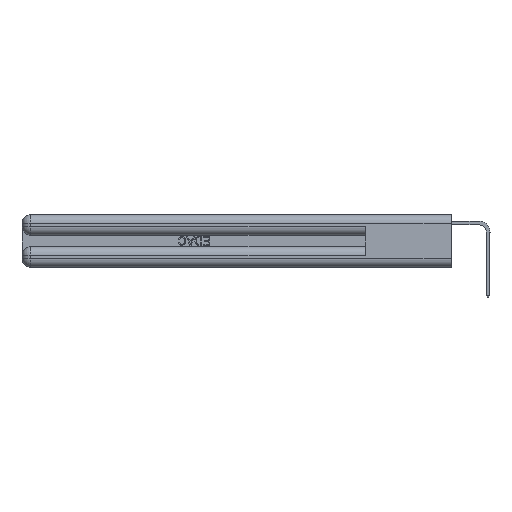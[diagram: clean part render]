
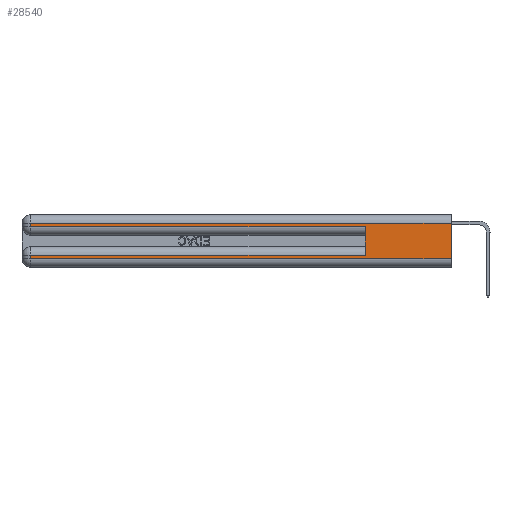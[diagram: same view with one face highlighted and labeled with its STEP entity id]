
A CAD part, left-side view. The second image highlights one B-rep face of the part: STEP entity #28540.
In plain terms, the highlighted planar face has unit normal (-1, 0, 0).
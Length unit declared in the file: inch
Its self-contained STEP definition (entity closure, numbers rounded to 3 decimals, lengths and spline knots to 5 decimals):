
#274 = DIRECTION ( 'NONE',  ( 0., 0., 1. ) ) ;
#744 = CARTESIAN_POINT ( 'NONE',  ( 0., 0., 0.06 ) ) ;
#1285 = EDGE_CURVE ( 'NONE', #16184, #5448, #23620, .T. ) ;
#1514 = LINE ( 'NONE', #28508, #15376 ) ;
#1540 = VECTOR ( 'NONE', #11069, 39.37008 ) ;
#1986 = VECTOR ( 'NONE', #16828, 39.37008 ) ;
#2475 = CARTESIAN_POINT ( 'NONE',  ( 0., 2.94, 0.37 ) ) ;
#2780 = CARTESIAN_POINT ( 'NONE',  ( 0., 0., 0.285 ) ) ;
#2801 = LINE ( 'NONE', #14213, #1986 ) ;
#3840 = LINE ( 'NONE', #744, #9959 ) ;
#4921 = LINE ( 'NONE', #2780, #11020 ) ;
#5448 = VERTEX_POINT ( 'NONE', #11649 ) ;
#5494 = ORIENTED_EDGE ( 'NONE', *, *, #7704, .F. ) ;
#5837 = ORIENTED_EDGE ( 'NONE', *, *, #15777, .T. ) ;
#6245 = VECTOR ( 'NONE', #274, 39.37008 ) ;
#6740 = CARTESIAN_POINT ( 'NONE',  ( 0., 2.94, 0.06 ) ) ;
#7704 = EDGE_CURVE ( 'NONE', #12056, #11255, #27055, .T. ) ;
#7740 = CARTESIAN_POINT ( 'NONE',  ( 0., 0., 0.06 ) ) ;
#8704 = EDGE_LOOP ( 'NONE', ( #22854, #11418, #31754, #29557, #5494, #16030, #5837, #33102 ) ) ;
#9628 = CARTESIAN_POINT ( 'NONE',  ( 0., 0.6, 0.085 ) ) ;
#9959 = VECTOR ( 'NONE', #31980, 39.37008 ) ;
#9967 = LINE ( 'NONE', #10106, #16083 ) ;
#10106 = CARTESIAN_POINT ( 'NONE',  ( 0., 0., 0.37 ) ) ;
#11020 = VECTOR ( 'NONE', #15751, 39.37008 ) ;
#11069 = DIRECTION ( 'NONE',  ( 0., 1., 0. ) ) ;
#11255 = VERTEX_POINT ( 'NONE', #16984 ) ;
#11418 = ORIENTED_EDGE ( 'NONE', *, *, #13657, .T. ) ;
#11555 = DIRECTION ( 'NONE',  ( 1., 0., 0. ) ) ;
#11649 = CARTESIAN_POINT ( 'NONE',  ( 0., 2.94, 0.285 ) ) ;
#12056 = VERTEX_POINT ( 'NONE', #9628 ) ;
#12891 = DIRECTION ( 'NONE',  ( 0., 1., 0. ) ) ;
#13207 = EDGE_CURVE ( 'NONE', #12056, #21928, #21544, .T. ) ;
#13657 = EDGE_CURVE ( 'NONE', #28747, #16184, #1514, .T. ) ;
#14213 = CARTESIAN_POINT ( 'NONE',  ( 0., 2.94, 0.37 ) ) ;
#14844 = CARTESIAN_POINT ( 'NONE',  ( 0., 0., 0.31 ) ) ;
#15127 = FACE_OUTER_BOUND ( 'NONE', #8704, .T. ) ;
#15376 = VECTOR ( 'NONE', #12891, 39.37008 ) ;
#15751 = DIRECTION ( 'NONE',  ( 0., -1., 0. ) ) ;
#15777 = EDGE_CURVE ( 'NONE', #21928, #31711, #2801, .T. ) ;
#16030 = ORIENTED_EDGE ( 'NONE', *, *, #13207, .T. ) ;
#16083 = VECTOR ( 'NONE', #30978, 39.37008 ) ;
#16184 = VERTEX_POINT ( 'NONE', #31416 ) ;
#16639 = AXIS2_PLACEMENT_3D ( 'NONE', #32317, #11555, #29804 ) ;
#16643 = VECTOR ( 'NONE', #25953, 39.37008 ) ;
#16828 = DIRECTION ( 'NONE',  ( 0., 0., -1. ) ) ;
#16984 = CARTESIAN_POINT ( 'NONE',  ( 0., 0.6, 0.285 ) ) ;
#18237 = EDGE_CURVE ( 'NONE', #31711, #30176, #3840, .T. ) ;
#21544 = LINE ( 'NONE', #29318, #1540 ) ;
#21928 = VERTEX_POINT ( 'NONE', #26257 ) ;
#22854 = ORIENTED_EDGE ( 'NONE', *, *, #32385, .F. ) ;
#23552 = CARTESIAN_POINT ( 'NONE',  ( 0., 0.6, 0.145 ) ) ;
#23620 = LINE ( 'NONE', #2475, #16643 ) ;
#23870 = EDGE_CURVE ( 'NONE', #5448, #11255, #4921, .T. ) ;
#25953 = DIRECTION ( 'NONE',  ( 0., 0., -1. ) ) ;
#26257 = CARTESIAN_POINT ( 'NONE',  ( 0., 2.94, 0.085 ) ) ;
#27055 = LINE ( 'NONE', #23552, #6245 ) ;
#27190 = PLANE ( 'NONE',  #16639 ) ;
#28508 = CARTESIAN_POINT ( 'NONE',  ( 0., 0., 0.31 ) ) ;
#28540 = ADVANCED_FACE ( 'NONE', ( #15127 ), #27190, .F. ) ;
#28747 = VERTEX_POINT ( 'NONE', #14844 ) ;
#29318 = CARTESIAN_POINT ( 'NONE',  ( 0., 0., 0.085 ) ) ;
#29557 = ORIENTED_EDGE ( 'NONE', *, *, #23870, .T. ) ;
#29804 = DIRECTION ( 'NONE',  ( 0., 0., -1. ) ) ;
#30176 = VERTEX_POINT ( 'NONE', #7740 ) ;
#30978 = DIRECTION ( 'NONE',  ( 0., 0., -1. ) ) ;
#31416 = CARTESIAN_POINT ( 'NONE',  ( 0., 2.94, 0.31 ) ) ;
#31711 = VERTEX_POINT ( 'NONE', #6740 ) ;
#31754 = ORIENTED_EDGE ( 'NONE', *, *, #1285, .T. ) ;
#31980 = DIRECTION ( 'NONE',  ( 0., -1., 0. ) ) ;
#32317 = CARTESIAN_POINT ( 'NONE',  ( 0., 0., 0.37 ) ) ;
#32385 = EDGE_CURVE ( 'NONE', #28747, #30176, #9967, .T. ) ;
#33102 = ORIENTED_EDGE ( 'NONE', *, *, #18237, .T. ) ;
